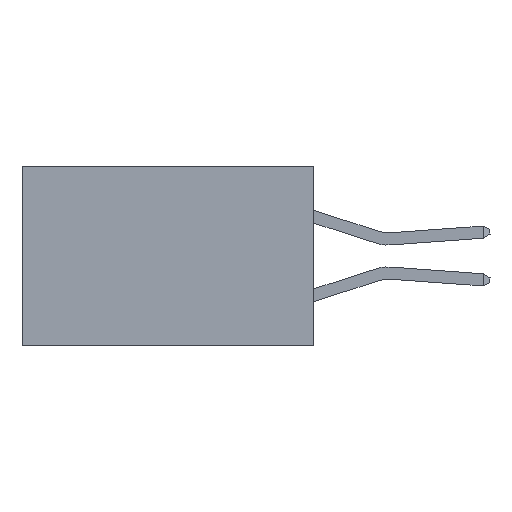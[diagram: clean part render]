
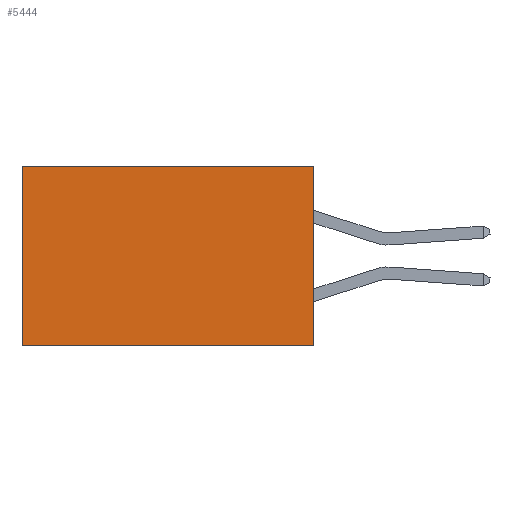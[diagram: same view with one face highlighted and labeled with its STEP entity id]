
A CAD part, left-side view. The second image highlights one B-rep face of the part: STEP entity #5444.
In plain terms, the highlighted planar face has unit normal (-1, 0, 0).
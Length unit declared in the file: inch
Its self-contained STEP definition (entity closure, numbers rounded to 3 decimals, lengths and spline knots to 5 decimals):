
#182 = VECTOR ( 'NONE', #47736, 39.37008 ) ;
#1666 = CARTESIAN_POINT ( 'NONE',  ( 0.2875, 0., 0. ) ) ;
#2763 = VECTOR ( 'NONE', #28025, 39.37008 ) ;
#5444 = ADVANCED_FACE ( 'NONE', ( #44637 ), #38461, .F. ) ;
#6792 = CARTESIAN_POINT ( 'NONE',  ( 0.2875, 0., 0. ) ) ;
#9039 = CARTESIAN_POINT ( 'NONE',  ( 0.2875, 0.6, 0. ) ) ;
#11771 = ORIENTED_EDGE ( 'NONE', *, *, #33774, .F. ) ;
#11970 = LINE ( 'NONE', #40156, #182 ) ;
#13477 = VERTEX_POINT ( 'NONE', #32160 ) ;
#13980 = AXIS2_PLACEMENT_3D ( 'NONE', #6792, #34320, #26054 ) ;
#16075 = VERTEX_POINT ( 'NONE', #9039 ) ;
#17069 = CARTESIAN_POINT ( 'NONE',  ( 0.2875, 0., 0. ) ) ;
#17507 = DIRECTION ( 'NONE',  ( 0., 1., 0. ) ) ;
#18461 = EDGE_CURVE ( 'NONE', #24072, #48570, #42176, .T. ) ;
#19198 = ORIENTED_EDGE ( 'NONE', *, *, #18461, .F. ) ;
#24072 = VERTEX_POINT ( 'NONE', #48486 ) ;
#25882 = LINE ( 'NONE', #42861, #26469 ) ;
#26054 = DIRECTION ( 'NONE',  ( 0., 0., -1. ) ) ;
#26469 = VECTOR ( 'NONE', #31117, 39.37008 ) ;
#28025 = DIRECTION ( 'NONE',  ( 0., 0., -1. ) ) ;
#29709 = EDGE_CURVE ( 'NONE', #16075, #13477, #25882, .T. ) ;
#30050 = VECTOR ( 'NONE', #17507, 39.37008 ) ;
#31117 = DIRECTION ( 'NONE',  ( 0., 0., -1. ) ) ;
#31402 = ORIENTED_EDGE ( 'NONE', *, *, #29709, .T. ) ;
#32160 = CARTESIAN_POINT ( 'NONE',  ( 0.2875, 0.6, -0.37 ) ) ;
#33774 = EDGE_CURVE ( 'NONE', #48570, #13477, #11970, .T. ) ;
#34320 = DIRECTION ( 'NONE',  ( 1., 0., 0. ) ) ;
#37149 = CARTESIAN_POINT ( 'NONE',  ( 0.2875, 0., -0.37 ) ) ;
#38461 = PLANE ( 'NONE',  #13980 ) ;
#40156 = CARTESIAN_POINT ( 'NONE',  ( 0.2875, 0., -0.37 ) ) ;
#42176 = LINE ( 'NONE', #17069, #2763 ) ;
#42861 = CARTESIAN_POINT ( 'NONE',  ( 0.2875, 0.6, 0. ) ) ;
#44637 = FACE_OUTER_BOUND ( 'NONE', #46238, .T. ) ;
#44856 = LINE ( 'NONE', #1666, #30050 ) ;
#46159 = ORIENTED_EDGE ( 'NONE', *, *, #49727, .T. ) ;
#46238 = EDGE_LOOP ( 'NONE', ( #31402, #11771, #19198, #46159 ) ) ;
#47736 = DIRECTION ( 'NONE',  ( 0., 1., 0. ) ) ;
#48486 = CARTESIAN_POINT ( 'NONE',  ( 0.2875, 0., 0. ) ) ;
#48570 = VERTEX_POINT ( 'NONE', #37149 ) ;
#49727 = EDGE_CURVE ( 'NONE', #24072, #16075, #44856, .T. ) ;
